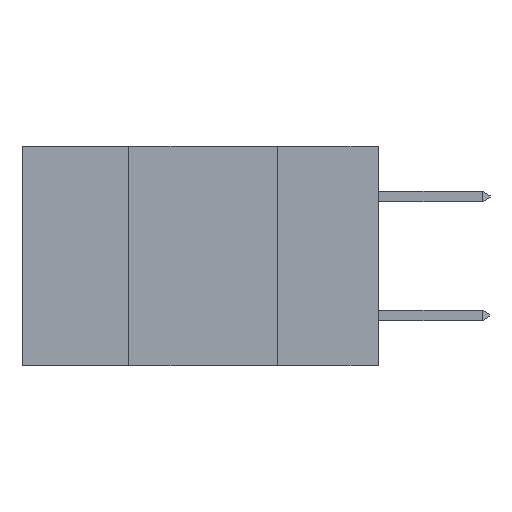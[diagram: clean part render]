
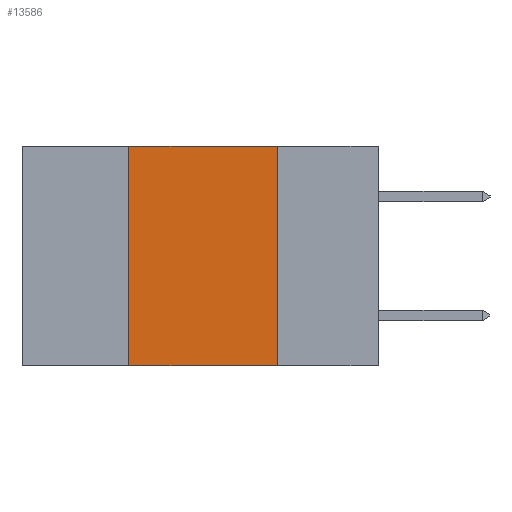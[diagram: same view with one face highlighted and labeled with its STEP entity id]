
A CAD part, left-side view. The second image highlights one B-rep face of the part: STEP entity #13586.
In plain terms, the highlighted planar face has unit normal (-1, 0, 0).
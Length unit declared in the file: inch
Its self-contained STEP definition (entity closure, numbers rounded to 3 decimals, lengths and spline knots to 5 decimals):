
#35 = VERTEX_POINT ( 'NONE', #4560 ) ;
#279 = VERTEX_POINT ( 'NONE', #12147 ) ;
#652 = LINE ( 'NONE', #11265, #10375 ) ;
#750 = VECTOR ( 'NONE', #5408, 39.37008 ) ;
#1226 = LINE ( 'NONE', #18750, #5555 ) ;
#1388 = ORIENTED_EDGE ( 'NONE', *, *, #14938, .T. ) ;
#1614 = EDGE_CURVE ( 'NONE', #279, #35, #15167, .T. ) ;
#2379 = CARTESIAN_POINT ( 'NONE',  ( 0., 0.6, -0.37 ) ) ;
#4075 = FACE_OUTER_BOUND ( 'NONE', #18818, .T. ) ;
#4382 = CARTESIAN_POINT ( 'NONE',  ( 0., 0.42, -0.37 ) ) ;
#4560 = CARTESIAN_POINT ( 'NONE',  ( 0., 0.42, 0. ) ) ;
#5408 = DIRECTION ( 'NONE',  ( 0., 0., 1. ) ) ;
#5555 = VECTOR ( 'NONE', #9828, 39.37008 ) ;
#5689 = AXIS2_PLACEMENT_3D ( 'NONE', #20530, #22275, #11713 ) ;
#5820 = DIRECTION ( 'NONE',  ( 0., -1., 0. ) ) ;
#6460 = CARTESIAN_POINT ( 'NONE',  ( 0., 0.17, 0. ) ) ;
#9718 = DIRECTION ( 'NONE',  ( 0., -1., 0. ) ) ;
#9828 = DIRECTION ( 'NONE',  ( 0., 0., -1. ) ) ;
#9955 = ORIENTED_EDGE ( 'NONE', *, *, #20118, .F. ) ;
#10375 = VECTOR ( 'NONE', #5820, 39.37008 ) ;
#10637 = EDGE_CURVE ( 'NONE', #17800, #11814, #1226, .T. ) ;
#11265 = CARTESIAN_POINT ( 'NONE',  ( 0., 0.6, 0. ) ) ;
#11713 = DIRECTION ( 'NONE',  ( 0., 0., -1. ) ) ;
#11814 = VERTEX_POINT ( 'NONE', #21977 ) ;
#12147 = CARTESIAN_POINT ( 'NONE',  ( 0., 0.42, -0.37 ) ) ;
#13544 = ORIENTED_EDGE ( 'NONE', *, *, #10637, .F. ) ;
#13586 = ADVANCED_FACE ( 'NONE', ( #4075 ), #18766, .F. ) ;
#14938 = EDGE_CURVE ( 'NONE', #279, #11814, #22400, .T. ) ;
#15167 = LINE ( 'NONE', #4382, #750 ) ;
#17749 = VECTOR ( 'NONE', #9718, 39.37008 ) ;
#17800 = VERTEX_POINT ( 'NONE', #6460 ) ;
#18750 = CARTESIAN_POINT ( 'NONE',  ( 0., 0.17, -0.37 ) ) ;
#18766 = PLANE ( 'NONE',  #5689 ) ;
#18818 = EDGE_LOOP ( 'NONE', ( #13544, #9955, #19927, #1388 ) ) ;
#19927 = ORIENTED_EDGE ( 'NONE', *, *, #1614, .F. ) ;
#20118 = EDGE_CURVE ( 'NONE', #35, #17800, #652, .T. ) ;
#20530 = CARTESIAN_POINT ( 'NONE',  ( 0., 0.6, 0. ) ) ;
#21977 = CARTESIAN_POINT ( 'NONE',  ( 0., 0.17, -0.37 ) ) ;
#22275 = DIRECTION ( 'NONE',  ( 1., 0., 0. ) ) ;
#22400 = LINE ( 'NONE', #2379, #17749 ) ;
